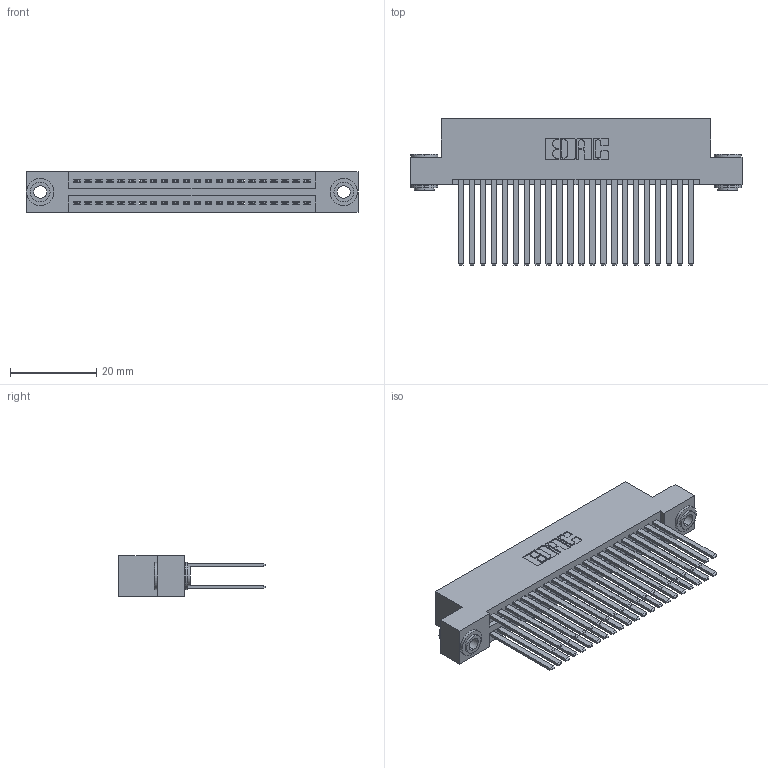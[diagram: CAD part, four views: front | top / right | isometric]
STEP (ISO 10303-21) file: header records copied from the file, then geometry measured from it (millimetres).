
FILE_DESCRIPTION (( 'STEP AP203' ), '1' );
FILE_NAME ('395-044-544-203.STEP', '2018-11-15T21:27:38', ( '' ), ( '' ), 'SwSTEP 2.0', 'SolidWorks 2016', '' );
FILE_SCHEMA (( 'CONFIG_CONTROL_DESIGN' ));
Length unit declared in the file: inch
Products named in the file (4): 345-250-002_345-250-002-102; 345 Part_Flush Mounting Lugs - 0.156 Dia-TH; 345-292-001_345-293-144; 395-044-544-203
Assembly tree (47 placements, depth 2):
  395-044-544-203
    345 Part_Flush Mounting Lugs - 0.156 Dia-TH
    345-292-001_345-293-144  x44
    345-250-002_345-250-002-102  x2
Bounding box: 77.09 x 33.96 x 9.4 mm (x, y, z)
Volume: 7939 mm3; surface area: 13360.6 mm2
Topology: 47 solids, 47 shells, 2100 faces, 6181 edges, 4058 vertices
Faces by surface type: plane 1366, cylinder 726, cone 8
Entity records: 20420 total; most frequent: CARTESIAN_POINT 3415, ORIENTED_EDGE 3342, DIRECTION 3065, EDGE_CURVE 1671, LINE 1431, VECTOR 1431, VERTEX_POINT 1110, AXIS2_PLACEMENT_3D 817
